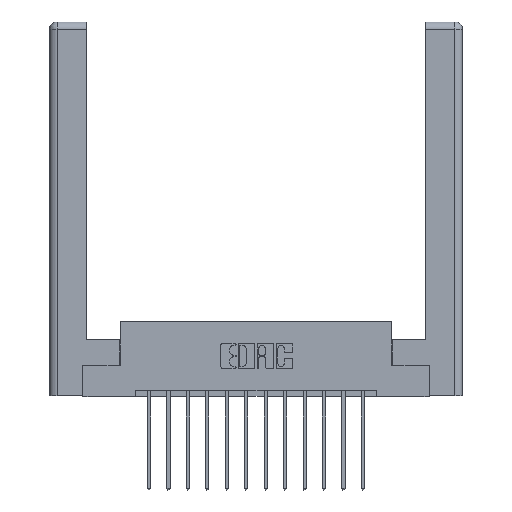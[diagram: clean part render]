
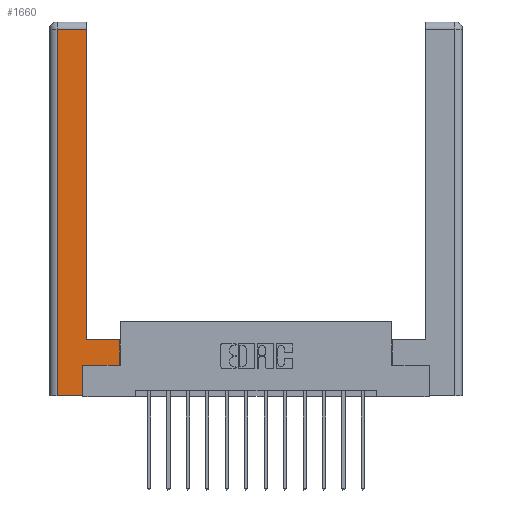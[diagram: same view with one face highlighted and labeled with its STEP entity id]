
A CAD part, top view. The second image highlights one B-rep face of the part: STEP entity #1660.
In plain terms, the highlighted planar face has unit normal (0, 0, 1).
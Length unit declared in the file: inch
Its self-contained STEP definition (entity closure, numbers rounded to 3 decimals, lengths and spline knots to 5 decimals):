
#80 = CARTESIAN_POINT ( 'NONE',  ( 0.0615, 2.94, 0. ) ) ;
#203 = VERTEX_POINT ( 'NONE', #1986 ) ;
#677 = CARTESIAN_POINT ( 'NONE',  ( 0.0615, 0., 0. ) ) ;
#836 = CARTESIAN_POINT ( 'NONE',  ( 0.295, 3., 0. ) ) ;
#1181 = DIRECTION ( 'NONE',  ( 1., 0., 0. ) ) ;
#1364 = AXIS2_PLACEMENT_3D ( 'NONE', #2084, #3322, #11914 ) ;
#1422 = CARTESIAN_POINT ( 'NONE',  ( 0.0615, 0., 0. ) ) ;
#1448 = LINE ( 'NONE', #2372, #14120 ) ;
#1498 = ORIENTED_EDGE ( 'NONE', *, *, #7804, .T. ) ;
#1660 = ADVANCED_FACE ( 'NONE', ( #3151 ), #9442, .F. ) ;
#1986 = CARTESIAN_POINT ( 'NONE',  ( 0.0615, 2.94, 0. ) ) ;
#2084 = CARTESIAN_POINT ( 'NONE',  ( 0., 0., 0. ) ) ;
#2220 = VECTOR ( 'NONE', #1181, 39.37008 ) ;
#2372 = CARTESIAN_POINT ( 'NONE',  ( 0.565, 0.245, 0. ) ) ;
#2535 = CARTESIAN_POINT ( 'NONE',  ( 0.265, 0.245, 0. ) ) ;
#2558 = EDGE_CURVE ( 'NONE', #5755, #4397, #6556, .T. ) ;
#2615 = LINE ( 'NONE', #12297, #2220 ) ;
#2783 = LINE ( 'NONE', #836, #13754 ) ;
#2894 = VECTOR ( 'NONE', #3757, 39.37008 ) ;
#2972 = CARTESIAN_POINT ( 'NONE',  ( 0.565, 0.245, 0. ) ) ;
#3099 = LINE ( 'NONE', #80, #2894 ) ;
#3151 = FACE_OUTER_BOUND ( 'NONE', #9214, .T. ) ;
#3322 = DIRECTION ( 'NONE',  ( 0., 0., -1. ) ) ;
#3344 = DIRECTION ( 'NONE',  ( 0., 1., 0. ) ) ;
#3410 = VERTEX_POINT ( 'NONE', #1422 ) ;
#3657 = DIRECTION ( 'NONE',  ( 1., 0., 0. ) ) ;
#3757 = DIRECTION ( 'NONE',  ( -1., 0., 0. ) ) ;
#4089 = CARTESIAN_POINT ( 'NONE',  ( 0.265, 0.245, 0. ) ) ;
#4114 = VECTOR ( 'NONE', #4889, 39.37008 ) ;
#4397 = VERTEX_POINT ( 'NONE', #14966 ) ;
#4889 = DIRECTION ( 'NONE',  ( -1., 0., 0. ) ) ;
#5179 = VERTEX_POINT ( 'NONE', #2972 ) ;
#5335 = ORIENTED_EDGE ( 'NONE', *, *, #11715, .T. ) ;
#5475 = EDGE_CURVE ( 'NONE', #203, #3410, #13873, .T. ) ;
#5722 = ORIENTED_EDGE ( 'NONE', *, *, #15715, .T. ) ;
#5736 = ORIENTED_EDGE ( 'NONE', *, *, #11276, .T. ) ;
#5755 = VERTEX_POINT ( 'NONE', #8364 ) ;
#5782 = CARTESIAN_POINT ( 'NONE',  ( 0.565, 0.45, 0. ) ) ;
#6507 = VECTOR ( 'NONE', #14286, 39.37008 ) ;
#6556 = LINE ( 'NONE', #11986, #4114 ) ;
#7239 = ORIENTED_EDGE ( 'NONE', *, *, #2558, .T. ) ;
#7804 = EDGE_CURVE ( 'NONE', #3410, #15133, #2615, .T. ) ;
#7888 = CARTESIAN_POINT ( 'NONE',  ( 0.295, 2.94, 0. ) ) ;
#8364 = CARTESIAN_POINT ( 'NONE',  ( 0.565, 0.45, 0. ) ) ;
#9171 = ORIENTED_EDGE ( 'NONE', *, *, #15083, .T. ) ;
#9211 = VERTEX_POINT ( 'NONE', #7888 ) ;
#9214 = EDGE_LOOP ( 'NONE', ( #5335, #9171, #11708, #1498, #5736, #10337, #5722, #7239 ) ) ;
#9442 = PLANE ( 'NONE',  #1364 ) ;
#9690 = LINE ( 'NONE', #2535, #12588 ) ;
#10211 = VECTOR ( 'NONE', #14148, 39.37008 ) ;
#10337 = ORIENTED_EDGE ( 'NONE', *, *, #11112, .T. ) ;
#11112 = EDGE_CURVE ( 'NONE', #15282, #5179, #1448, .T. ) ;
#11276 = EDGE_CURVE ( 'NONE', #15133, #15282, #9690, .T. ) ;
#11708 = ORIENTED_EDGE ( 'NONE', *, *, #5475, .T. ) ;
#11715 = EDGE_CURVE ( 'NONE', #4397, #9211, #2783, .T. ) ;
#11914 = DIRECTION ( 'NONE',  ( -1., 0., 0. ) ) ;
#11986 = CARTESIAN_POINT ( 'NONE',  ( 0.295, 0.45, 0. ) ) ;
#12297 = CARTESIAN_POINT ( 'NONE',  ( 0.265, 0., 0. ) ) ;
#12588 = VECTOR ( 'NONE', #13554, 39.37008 ) ;
#12695 = LINE ( 'NONE', #5782, #6507 ) ;
#13554 = DIRECTION ( 'NONE',  ( 0., 1., 0. ) ) ;
#13754 = VECTOR ( 'NONE', #3344, 39.37008 ) ;
#13873 = LINE ( 'NONE', #677, #10211 ) ;
#14120 = VECTOR ( 'NONE', #3657, 39.37008 ) ;
#14148 = DIRECTION ( 'NONE',  ( 0., -1., 0. ) ) ;
#14286 = DIRECTION ( 'NONE',  ( 0., 1., 0. ) ) ;
#14635 = CARTESIAN_POINT ( 'NONE',  ( 0.265, 0., 0. ) ) ;
#14966 = CARTESIAN_POINT ( 'NONE',  ( 0.295, 0.45, 0. ) ) ;
#15083 = EDGE_CURVE ( 'NONE', #9211, #203, #3099, .T. ) ;
#15133 = VERTEX_POINT ( 'NONE', #14635 ) ;
#15282 = VERTEX_POINT ( 'NONE', #4089 ) ;
#15715 = EDGE_CURVE ( 'NONE', #5179, #5755, #12695, .T. ) ;
